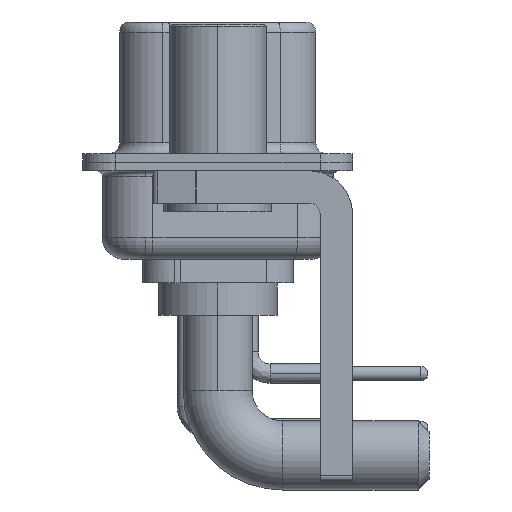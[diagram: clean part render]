
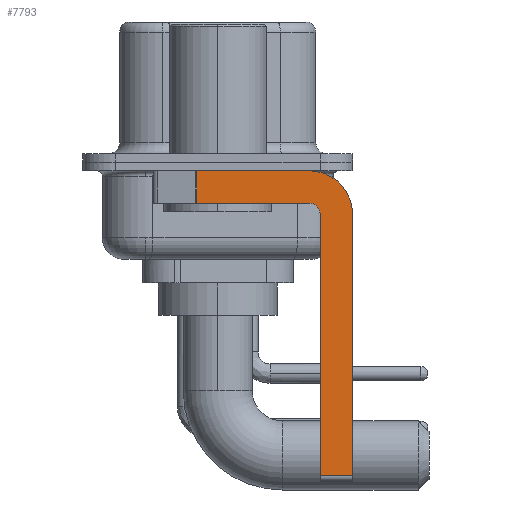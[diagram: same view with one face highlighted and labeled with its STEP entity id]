
A CAD part, left-side view. The second image highlights one B-rep face of the part: STEP entity #7793.
In plain terms, the highlighted planar face has unit normal (-1, 0, 0).
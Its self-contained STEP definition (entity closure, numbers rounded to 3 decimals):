
#132 = ORIENTED_EDGE ( 'NONE', *, *, #18231, .T. ) ;
#240 = CARTESIAN_POINT ( 'NONE',  ( -2.9, 3., -0.4 ) ) ;
#409 = ORIENTED_EDGE ( 'NONE', *, *, #5499, .F. ) ;
#1144 = CARTESIAN_POINT ( 'NONE',  ( -2.9, -4.25, -1.9 ) ) ;
#1661 = CARTESIAN_POINT ( 'NONE',  ( -2.9, -4.25, -2.4 ) ) ;
#1725 = CARTESIAN_POINT ( 'NONE',  ( -2.9, 0.978, -1.9 ) ) ;
#1839 = DIRECTION ( 'NONE',  ( 0., 0., 1. ) ) ;
#2487 = LINE ( 'NONE', #19307, #18068 ) ;
#2745 = EDGE_LOOP ( 'NONE', ( #13668, #132, #12514, #24115, #409, #11991, #5064, #18675 ) ) ;
#2808 = DIRECTION ( 'NONE',  ( 0., -1., 0. ) ) ;
#3465 = EDGE_CURVE ( 'NONE', #11269, #7789, #13695, .T. ) ;
#4635 = CARTESIAN_POINT ( 'NONE',  ( -2.9, -4.25, -14.55 ) ) ;
#5064 = ORIENTED_EDGE ( 'NONE', *, *, #23566, .F. ) ;
#5162 = CIRCLE ( 'NONE', #14830, 0.5 ) ;
#5175 = CARTESIAN_POINT ( 'NONE',  ( -2.9, -4.25, -1.9 ) ) ;
#5245 = EDGE_CURVE ( 'NONE', #18727, #17372, #5162, .T. ) ;
#5273 = CARTESIAN_POINT ( 'NONE',  ( -2.9, -4.25, -0.4 ) ) ;
#5392 = VECTOR ( 'NONE', #7642, 1000. ) ;
#5499 = EDGE_CURVE ( 'NONE', #24938, #18727, #17273, .T. ) ;
#6768 = DIRECTION ( 'NONE',  ( 0., 0., -1. ) ) ;
#7109 = EDGE_CURVE ( 'NONE', #17372, #16759, #15478, .T. ) ;
#7123 = DIRECTION ( 'NONE',  ( 1., 0., 0. ) ) ;
#7642 = DIRECTION ( 'NONE',  ( 0., 1., 0. ) ) ;
#7789 = VERTEX_POINT ( 'NONE', #14475 ) ;
#7793 = ADVANCED_FACE ( 'NONE', ( #18215 ), #22882, .F. ) ;
#8075 = VECTOR ( 'NONE', #11703, 1000. ) ;
#9051 = CARTESIAN_POINT ( 'NONE',  ( -2.9, -4.75, -2.4 ) ) ;
#10094 = DIRECTION ( 'NONE',  ( 0., 0., -1. ) ) ;
#10150 = CARTESIAN_POINT ( 'NONE',  ( -2.9, 0.978, -0.4 ) ) ;
#10645 = AXIS2_PLACEMENT_3D ( 'NONE', #17598, #7123, #11406 ) ;
#10742 = LINE ( 'NONE', #240, #22322 ) ;
#11269 = VERTEX_POINT ( 'NONE', #5273 ) ;
#11406 = DIRECTION ( 'NONE',  ( 0., 0., -1. ) ) ;
#11703 = DIRECTION ( 'NONE',  ( 0., 0., -1. ) ) ;
#11927 = CARTESIAN_POINT ( 'NONE',  ( -2.9, -4.25, -2.4 ) ) ;
#11991 = ORIENTED_EDGE ( 'NONE', *, *, #17334, .T. ) ;
#12410 = AXIS2_PLACEMENT_3D ( 'NONE', #1661, #18748, #10094 ) ;
#12471 = DIRECTION ( 'NONE',  ( 0., 0., 1. ) ) ;
#12514 = ORIENTED_EDGE ( 'NONE', *, *, #7109, .F. ) ;
#12734 = CARTESIAN_POINT ( 'NONE',  ( -2.9, -4.75, -14.8 ) ) ;
#13269 = EDGE_CURVE ( 'NONE', #18874, #11269, #10742, .T. ) ;
#13668 = ORIENTED_EDGE ( 'NONE', *, *, #13269, .F. ) ;
#13695 = CIRCLE ( 'NONE', #10645, 2. ) ;
#14475 = CARTESIAN_POINT ( 'NONE',  ( -2.9, -6.25, -2.4 ) ) ;
#14591 = DIRECTION ( 'NONE',  ( 0., -1., 0. ) ) ;
#14830 = AXIS2_PLACEMENT_3D ( 'NONE', #11927, #24871, #1839 ) ;
#15478 = LINE ( 'NONE', #1144, #5392 ) ;
#15546 = CARTESIAN_POINT ( 'NONE',  ( -2.9, -6.25, -2.4 ) ) ;
#16179 = CARTESIAN_POINT ( 'NONE',  ( -2.9, -4.75, -14.55 ) ) ;
#16694 = VECTOR ( 'NONE', #2808, 1000. ) ;
#16759 = VERTEX_POINT ( 'NONE', #1725 ) ;
#17273 = LINE ( 'NONE', #12734, #21872 ) ;
#17334 = EDGE_CURVE ( 'NONE', #24938, #20690, #17570, .T. ) ;
#17372 = VERTEX_POINT ( 'NONE', #5175 ) ;
#17570 = LINE ( 'NONE', #4635, #16694 ) ;
#17598 = CARTESIAN_POINT ( 'NONE',  ( -2.9, -4.25, -2.4 ) ) ;
#18068 = VECTOR ( 'NONE', #6768, 1000. ) ;
#18215 = FACE_OUTER_BOUND ( 'NONE', #2745, .T. ) ;
#18231 = EDGE_CURVE ( 'NONE', #18874, #16759, #2487, .T. ) ;
#18675 = ORIENTED_EDGE ( 'NONE', *, *, #3465, .F. ) ;
#18727 = VERTEX_POINT ( 'NONE', #9051 ) ;
#18748 = DIRECTION ( 'NONE',  ( 1., 0., 0. ) ) ;
#18874 = VERTEX_POINT ( 'NONE', #10150 ) ;
#19307 = CARTESIAN_POINT ( 'NONE',  ( -2.9, 0.978, -1.9 ) ) ;
#20690 = VERTEX_POINT ( 'NONE', #21742 ) ;
#21742 = CARTESIAN_POINT ( 'NONE',  ( -2.9, -6.25, -14.55 ) ) ;
#21872 = VECTOR ( 'NONE', #12471, 1000. ) ;
#22322 = VECTOR ( 'NONE', #14591, 1000. ) ;
#22882 = PLANE ( 'NONE',  #12410 ) ;
#23566 = EDGE_CURVE ( 'NONE', #7789, #20690, #26446, .T. ) ;
#24115 = ORIENTED_EDGE ( 'NONE', *, *, #5245, .F. ) ;
#24871 = DIRECTION ( 'NONE',  ( -1., 0., 0. ) ) ;
#24938 = VERTEX_POINT ( 'NONE', #16179 ) ;
#26446 = LINE ( 'NONE', #15546, #8075 ) ;
